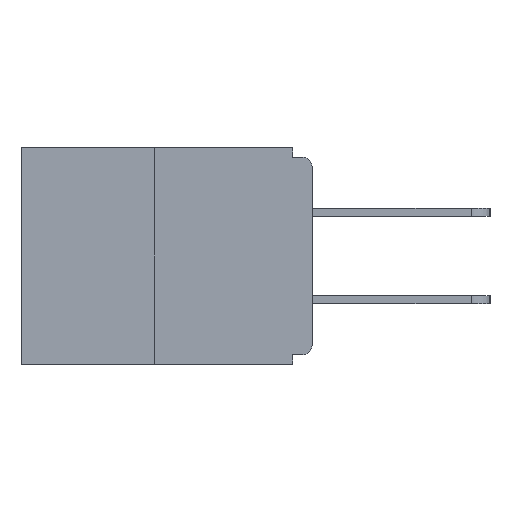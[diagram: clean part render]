
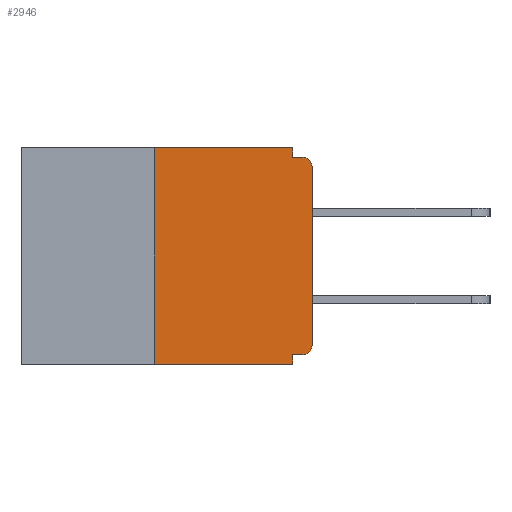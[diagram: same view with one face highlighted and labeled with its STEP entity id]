
A CAD part, left-side view. The second image highlights one B-rep face of the part: STEP entity #2946.
In plain terms, the highlighted planar face has unit normal (-1, 0, 0).
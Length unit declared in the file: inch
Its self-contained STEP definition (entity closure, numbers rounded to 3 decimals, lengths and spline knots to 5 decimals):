
#263 = PLANE ( 'NONE',  #5693 ) ;
#1554 = VERTEX_POINT ( 'NONE', #28072 ) ;
#1596 = EDGE_CURVE ( 'NONE', #1554, #28490, #21806, .T. ) ;
#2249 = CIRCLE ( 'NONE', #4659, 0.015 ) ;
#2298 = CARTESIAN_POINT ( 'NONE',  ( 0., 0., -0.313 ) ) ;
#2668 = VERTEX_POINT ( 'NONE', #21533 ) ;
#2946 = ADVANCED_FACE ( 'NONE', ( #15031 ), #263, .F. ) ;
#3026 = VECTOR ( 'NONE', #15691, 39.37008 ) ;
#4400 = AXIS2_PLACEMENT_3D ( 'NONE', #20570, #7148, #7636 ) ;
#4581 = DIRECTION ( 'NONE',  ( 0., 0., 1. ) ) ;
#4659 = AXIS2_PLACEMENT_3D ( 'NONE', #4709, #20417, #16006 ) ;
#4709 = CARTESIAN_POINT ( 'NONE',  ( 0., 0.015, -0.03 ) ) ;
#5072 = DIRECTION ( 'NONE',  ( 0., 0., -1. ) ) ;
#5306 = CARTESIAN_POINT ( 'NONE',  ( 0., 0.031, -0.343 ) ) ;
#5416 = CARTESIAN_POINT ( 'NONE',  ( 0., 0.25, -0.343 ) ) ;
#5632 = ORIENTED_EDGE ( 'NONE', *, *, #14229, .T. ) ;
#5646 = ORIENTED_EDGE ( 'NONE', *, *, #28871, .F. ) ;
#5693 = AXIS2_PLACEMENT_3D ( 'NONE', #7073, #15987, #5072 ) ;
#5825 = EDGE_CURVE ( 'NONE', #10438, #28490, #14587, .T. ) ;
#6125 = CARTESIAN_POINT ( 'NONE',  ( 0., 0., 0. ) ) ;
#6257 = VERTEX_POINT ( 'NONE', #21331 ) ;
#6304 = EDGE_CURVE ( 'NONE', #22790, #14829, #9309, .T. ) ;
#6838 = CARTESIAN_POINT ( 'NONE',  ( 0., 0.015, -0.015 ) ) ;
#7073 = CARTESIAN_POINT ( 'NONE',  ( 0., 0.46, 0. ) ) ;
#7148 = DIRECTION ( 'NONE',  ( -1., 0., 0. ) ) ;
#7636 = DIRECTION ( 'NONE',  ( 0., 0., -1. ) ) ;
#8206 = CARTESIAN_POINT ( 'NONE',  ( 0., 0.46, -0.343 ) ) ;
#8721 = CARTESIAN_POINT ( 'NONE',  ( 0., 0.031, 0. ) ) ;
#9176 = EDGE_CURVE ( 'NONE', #21430, #1554, #25394, .T. ) ;
#9309 = LINE ( 'NONE', #6125, #14560 ) ;
#9456 = CARTESIAN_POINT ( 'NONE',  ( 0., 0., -0.328 ) ) ;
#9541 = ORIENTED_EDGE ( 'NONE', *, *, #6304, .T. ) ;
#9935 = ORIENTED_EDGE ( 'NONE', *, *, #18001, .T. ) ;
#10219 = CARTESIAN_POINT ( 'NONE',  ( 0., 0.031, -0.343 ) ) ;
#10289 = ORIENTED_EDGE ( 'NONE', *, *, #27698, .F. ) ;
#10438 = VERTEX_POINT ( 'NONE', #5416 ) ;
#11370 = ORIENTED_EDGE ( 'NONE', *, *, #1596, .F. ) ;
#12887 = LINE ( 'NONE', #24144, #28066 ) ;
#13346 = VECTOR ( 'NONE', #19369, 39.37008 ) ;
#13498 = CARTESIAN_POINT ( 'NONE',  ( 0., 0., -0.03 ) ) ;
#13630 = DIRECTION ( 'NONE',  ( 0., -1., 0. ) ) ;
#14229 = EDGE_CURVE ( 'NONE', #21430, #22790, #28063, .T. ) ;
#14239 = DIRECTION ( 'NONE',  ( 0., 1., 0. ) ) ;
#14560 = VECTOR ( 'NONE', #22123, 39.37008 ) ;
#14587 = LINE ( 'NONE', #8206, #19532 ) ;
#14829 = VERTEX_POINT ( 'NONE', #13498 ) ;
#15031 = FACE_OUTER_BOUND ( 'NONE', #19355, .T. ) ;
#15691 = DIRECTION ( 'NONE',  ( 0., 0., -1. ) ) ;
#15752 = VECTOR ( 'NONE', #13630, 39.37008 ) ;
#15987 = DIRECTION ( 'NONE',  ( 1., 0., 0. ) ) ;
#16006 = DIRECTION ( 'NONE',  ( 0., 0., -1. ) ) ;
#16053 = LINE ( 'NONE', #24761, #21309 ) ;
#16796 = ORIENTED_EDGE ( 'NONE', *, *, #9176, .F. ) ;
#17430 = DIRECTION ( 'NONE',  ( 0., -1., 0. ) ) ;
#17769 = CARTESIAN_POINT ( 'NONE',  ( 0., 0.015, -0.328 ) ) ;
#18001 = EDGE_CURVE ( 'NONE', #14829, #22827, #2249, .T. ) ;
#18359 = ORIENTED_EDGE ( 'NONE', *, *, #5825, .T. ) ;
#18679 = VECTOR ( 'NONE', #14239, 39.37008 ) ;
#19355 = EDGE_LOOP ( 'NONE', ( #10289, #22794, #18359, #11370, #16796, #5632, #9541, #9935, #24598, #5646 ) ) ;
#19369 = DIRECTION ( 'NONE',  ( 0., 0., -1. ) ) ;
#19391 = DIRECTION ( 'NONE',  ( 0., -1., 0. ) ) ;
#19532 = VECTOR ( 'NONE', #19391, 39.37008 ) ;
#20417 = DIRECTION ( 'NONE',  ( -1., 0., 0. ) ) ;
#20570 = CARTESIAN_POINT ( 'NONE',  ( 0., 0.015, -0.313 ) ) ;
#21309 = VECTOR ( 'NONE', #4581, 39.37008 ) ;
#21331 = CARTESIAN_POINT ( 'NONE',  ( 0., 0.031, -0.015 ) ) ;
#21334 = EDGE_CURVE ( 'NONE', #6257, #22827, #27750, .T. ) ;
#21430 = VERTEX_POINT ( 'NONE', #17769 ) ;
#21533 = CARTESIAN_POINT ( 'NONE',  ( 0., 0.031, 0. ) ) ;
#21806 = LINE ( 'NONE', #10219, #13346 ) ;
#21982 = LINE ( 'NONE', #8721, #3026 ) ;
#22123 = DIRECTION ( 'NONE',  ( 0., 0., 1. ) ) ;
#22594 = EDGE_CURVE ( 'NONE', #10438, #23641, #16053, .T. ) ;
#22790 = VERTEX_POINT ( 'NONE', #2298 ) ;
#22794 = ORIENTED_EDGE ( 'NONE', *, *, #22594, .F. ) ;
#22827 = VERTEX_POINT ( 'NONE', #6838 ) ;
#23641 = VERTEX_POINT ( 'NONE', #27354 ) ;
#24144 = CARTESIAN_POINT ( 'NONE',  ( 0., 0.46, 0. ) ) ;
#24598 = ORIENTED_EDGE ( 'NONE', *, *, #21334, .F. ) ;
#24761 = CARTESIAN_POINT ( 'NONE',  ( 0., 0.25, 0. ) ) ;
#25394 = LINE ( 'NONE', #9456, #18679 ) ;
#27153 = CARTESIAN_POINT ( 'NONE',  ( 0., 0., -0.015 ) ) ;
#27354 = CARTESIAN_POINT ( 'NONE',  ( 0., 0.25, 0. ) ) ;
#27698 = EDGE_CURVE ( 'NONE', #23641, #2668, #12887, .T. ) ;
#27750 = LINE ( 'NONE', #27153, #15752 ) ;
#28063 = CIRCLE ( 'NONE', #4400, 0.015 ) ;
#28066 = VECTOR ( 'NONE', #17430, 39.37008 ) ;
#28072 = CARTESIAN_POINT ( 'NONE',  ( 0., 0.031, -0.328 ) ) ;
#28490 = VERTEX_POINT ( 'NONE', #5306 ) ;
#28871 = EDGE_CURVE ( 'NONE', #2668, #6257, #21982, .T. ) ;
